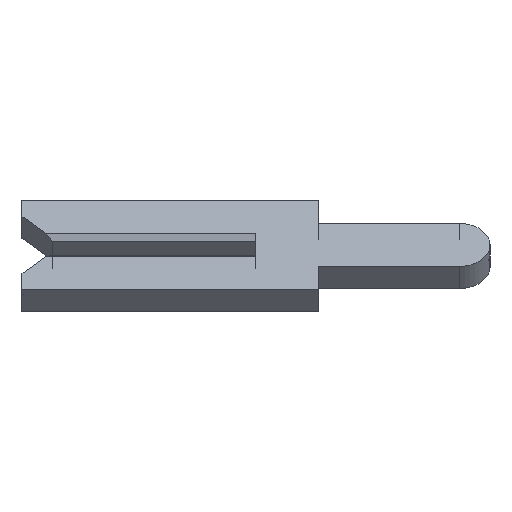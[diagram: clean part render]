
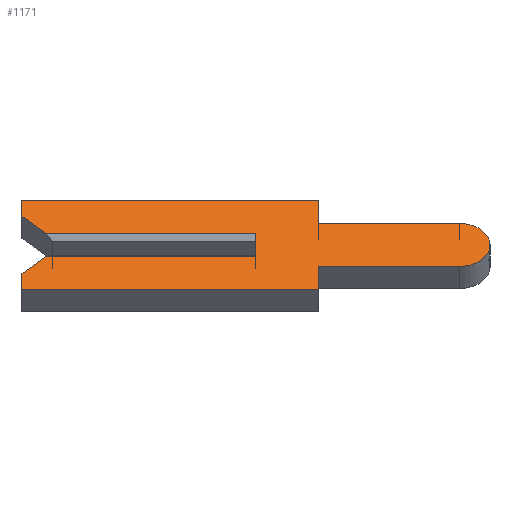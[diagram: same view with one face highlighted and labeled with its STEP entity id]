
A CAD part, left-side view. The second image highlights one B-rep face of the part: STEP entity #1171.
In plain terms, the highlighted face is planar.
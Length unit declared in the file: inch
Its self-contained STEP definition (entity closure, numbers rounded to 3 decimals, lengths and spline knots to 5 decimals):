
#3 = ORIENTED_EDGE ( 'NONE', *, *, #1020, .F. ) ;
#10 = ORIENTED_EDGE ( 'NONE', *, *, #328, .F. ) ;
#18 = DIRECTION ( 'NONE',  ( 0., -1., 0. ) ) ;
#20 = DIRECTION ( 'NONE',  ( 1., 0., 0. ) ) ;
#31 = VERTEX_POINT ( 'NONE', #914 ) ;
#44 = VECTOR ( 'NONE', #275, 39.37008 ) ;
#67 = LINE ( 'NONE', #552, #1460 ) ;
#86 = EDGE_CURVE ( 'NONE', #1322, #1650, #1158, .T. ) ;
#87 = CARTESIAN_POINT ( 'NONE',  ( -0.01, 0.15, 0.026 ) ) ;
#113 = EDGE_CURVE ( 'NONE', #359, #130, #922, .T. ) ;
#117 = VECTOR ( 'NONE', #1124, 39.37008 ) ;
#120 = VERTEX_POINT ( 'NONE', #534 ) ;
#130 = VERTEX_POINT ( 'NONE', #294 ) ;
#133 = VECTOR ( 'NONE', #931, 39.37008 ) ;
#145 = CARTESIAN_POINT ( 'NONE',  ( -0.01, 0.134, 0.01 ) ) ;
#149 = VECTOR ( 'NONE', #1108, 39.37008 ) ;
#172 = EDGE_CURVE ( 'NONE', #1380, #1164, #1426, .T. ) ;
#205 = EDGE_CURVE ( 'NONE', #312, #31, #1384, .T. ) ;
#230 = CARTESIAN_POINT ( 'NONE',  ( -0.01, 0.15, -0.04 ) ) ;
#275 = DIRECTION ( 'NONE',  ( 0., -1., 0. ) ) ;
#278 = DIRECTION ( 'NONE',  ( 0., 1., 0. ) ) ;
#294 = CARTESIAN_POINT ( 'NONE',  ( -0.01, 0., 0.01 ) ) ;
#312 = VERTEX_POINT ( 'NONE', #817 ) ;
#321 = VERTEX_POINT ( 'NONE', #949 ) ;
#328 = EDGE_CURVE ( 'NONE', #120, #1322, #1516, .T. ) ;
#333 = CARTESIAN_POINT ( 'NONE',  ( -0.01, 0.15, -0.026 ) ) ;
#359 = VERTEX_POINT ( 'NONE', #1584 ) ;
#383 = ORIENTED_EDGE ( 'NONE', *, *, #205, .F. ) ;
#388 = VECTOR ( 'NONE', #645, 39.37008 ) ;
#397 = AXIS2_PLACEMENT_3D ( 'NONE', #1318, #20, #1448 ) ;
#407 = EDGE_LOOP ( 'NONE', ( #1357, #1593, #838, #383, #664, #3, #1334, #567, #10, #1522, #1565, #471, #1489, #836 ) ) ;
#413 = CARTESIAN_POINT ( 'NONE',  ( -0.01, 0., 0.0065 ) ) ;
#426 = VECTOR ( 'NONE', #1528, 39.37008 ) ;
#471 = ORIENTED_EDGE ( 'NONE', *, *, #1507, .F. ) ;
#488 = CARTESIAN_POINT ( 'NONE',  ( -0.01, 0.1305, 0.0065 ) ) ;
#534 = CARTESIAN_POINT ( 'NONE',  ( -0.01, -0.1305, 0.0195 ) ) ;
#552 = CARTESIAN_POINT ( 'NONE',  ( -0.01, 0.15, 0.04 ) ) ;
#558 = EDGE_CURVE ( 'NONE', #1067, #312, #950, .T. ) ;
#567 = ORIENTED_EDGE ( 'NONE', *, *, #86, .F. ) ;
#627 = CARTESIAN_POINT ( 'NONE',  ( -0.01, 0.15, -0.04 ) ) ;
#645 = DIRECTION ( 'NONE',  ( 0., -1., 0. ) ) ;
#659 = CARTESIAN_POINT ( 'NONE',  ( -0.01, -0.04, 0.0195 ) ) ;
#664 = ORIENTED_EDGE ( 'NONE', *, *, #558, .F. ) ;
#671 = CARTESIAN_POINT ( 'NONE',  ( -0.01, -0.04, -0.04 ) ) ;
#684 = CARTESIAN_POINT ( 'NONE',  ( -0.01, -0.04, -0.04 ) ) ;
#731 = DIRECTION ( 'NONE',  ( 0., 0., 1. ) ) ;
#784 = DIRECTION ( 'NONE',  ( 0., 0., -1. ) ) ;
#789 = CARTESIAN_POINT ( 'NONE',  ( -0.01, 0.15, 0.04 ) ) ;
#790 = VECTOR ( 'NONE', #1268, 39.37008 ) ;
#791 = CARTESIAN_POINT ( 'NONE',  ( -0.01, -0.04, -0.0195 ) ) ;
#807 = DIRECTION ( 'NONE',  ( 0., 0., -1. ) ) ;
#816 = VECTOR ( 'NONE', #1430, 39.37008 ) ;
#817 = CARTESIAN_POINT ( 'NONE',  ( -0.01, 0.15, -0.026 ) ) ;
#818 = LINE ( 'NONE', #488, #790 ) ;
#836 = ORIENTED_EDGE ( 'NONE', *, *, #1204, .F. ) ;
#838 = ORIENTED_EDGE ( 'NONE', *, *, #1181, .F. ) ;
#879 = EDGE_CURVE ( 'NONE', #321, #1301, #1296, .T. ) ;
#914 = CARTESIAN_POINT ( 'NONE',  ( -0.01, 0.134, -0.01 ) ) ;
#922 = LINE ( 'NONE', #413, #816 ) ;
#931 = DIRECTION ( 'NONE',  ( 0., -0.707, 0.707 ) ) ;
#943 = CARTESIAN_POINT ( 'NONE',  ( -0.01, -0.04, 0.04 ) ) ;
#949 = CARTESIAN_POINT ( 'NONE',  ( -0.01, 0.15, 0.026 ) ) ;
#950 = LINE ( 'NONE', #333, #1250 ) ;
#955 = DIRECTION ( 'NONE',  ( 0., 0., -1. ) ) ;
#964 = LINE ( 'NONE', #659, #426 ) ;
#1002 = LINE ( 'NONE', #671, #1118 ) ;
#1017 = CARTESIAN_POINT ( 'NONE',  ( -0.01, -0.04, 0.0195 ) ) ;
#1020 = EDGE_CURVE ( 'NONE', #1572, #1067, #1327, .T. ) ;
#1023 = CARTESIAN_POINT ( 'NONE',  ( -0.01, -0.1305, -0.01 ) ) ;
#1054 = CARTESIAN_POINT ( 'NONE',  ( -0.01, -0.04, 0.04 ) ) ;
#1060 = LINE ( 'NONE', #1023, #388 ) ;
#1067 = VERTEX_POINT ( 'NONE', #627 ) ;
#1106 = AXIS2_PLACEMENT_3D ( 'NONE', #1419, #1403, #784 ) ;
#1108 = DIRECTION ( 'NONE',  ( 0., 0., 1. ) ) ;
#1118 = VECTOR ( 'NONE', #807, 39.37008 ) ;
#1124 = DIRECTION ( 'NONE',  ( 0., 1., 0. ) ) ;
#1127 = EDGE_CURVE ( 'NONE', #1164, #120, #964, .T. ) ;
#1147 = PLANE ( 'NONE',  #1106 ) ;
#1158 = LINE ( 'NONE', #791, #1603 ) ;
#1164 = VERTEX_POINT ( 'NONE', #1017 ) ;
#1171 = ADVANCED_FACE ( 'NONE', ( #1280 ), #1147, .F. ) ;
#1181 = EDGE_CURVE ( 'NONE', #31, #359, #1060, .T. ) ;
#1204 = EDGE_CURVE ( 'NONE', #1500, #321, #818, .T. ) ;
#1250 = VECTOR ( 'NONE', #731, 39.37008 ) ;
#1268 = DIRECTION ( 'NONE',  ( 0., 0.707, 0.707 ) ) ;
#1280 = FACE_OUTER_BOUND ( 'NONE', #407, .T. ) ;
#1296 = LINE ( 'NONE', #87, #149 ) ;
#1301 = VERTEX_POINT ( 'NONE', #789 ) ;
#1309 = CARTESIAN_POINT ( 'NONE',  ( -0.01, 0.15, 0.01 ) ) ;
#1318 = CARTESIAN_POINT ( 'NONE',  ( -0.01, -0.1305, 0. ) ) ;
#1322 = VERTEX_POINT ( 'NONE', #1413 ) ;
#1327 = LINE ( 'NONE', #230, #117 ) ;
#1334 = ORIENTED_EDGE ( 'NONE', *, *, #1560, .F. ) ;
#1357 = ORIENTED_EDGE ( 'NONE', *, *, #1423, .T. ) ;
#1380 = VERTEX_POINT ( 'NONE', #1054 ) ;
#1384 = LINE ( 'NONE', #1580, #133 ) ;
#1403 = DIRECTION ( 'NONE',  ( 1., 0., 0. ) ) ;
#1413 = CARTESIAN_POINT ( 'NONE',  ( -0.01, -0.1305, -0.0195 ) ) ;
#1419 = CARTESIAN_POINT ( 'NONE',  ( -0.01, -0.1305, 0. ) ) ;
#1423 = EDGE_CURVE ( 'NONE', #1500, #130, #1546, .T. ) ;
#1426 = LINE ( 'NONE', #943, #1566 ) ;
#1430 = DIRECTION ( 'NONE',  ( 0., 0., 1. ) ) ;
#1448 = DIRECTION ( 'NONE',  ( 0., 0., -1. ) ) ;
#1460 = VECTOR ( 'NONE', #18, 39.37008 ) ;
#1489 = ORIENTED_EDGE ( 'NONE', *, *, #879, .F. ) ;
#1500 = VERTEX_POINT ( 'NONE', #145 ) ;
#1507 = EDGE_CURVE ( 'NONE', #1301, #1380, #67, .T. ) ;
#1516 = CIRCLE ( 'NONE', #397, 0.0195 ) ;
#1522 = ORIENTED_EDGE ( 'NONE', *, *, #1127, .F. ) ;
#1528 = DIRECTION ( 'NONE',  ( 0., -1., 0. ) ) ;
#1546 = LINE ( 'NONE', #1309, #44 ) ;
#1560 = EDGE_CURVE ( 'NONE', #1650, #1572, #1002, .T. ) ;
#1565 = ORIENTED_EDGE ( 'NONE', *, *, #172, .F. ) ;
#1566 = VECTOR ( 'NONE', #955, 39.37008 ) ;
#1572 = VERTEX_POINT ( 'NONE', #684 ) ;
#1580 = CARTESIAN_POINT ( 'NONE',  ( -0.01, 0.1305, -0.0065 ) ) ;
#1584 = CARTESIAN_POINT ( 'NONE',  ( -0.01, 0., -0.01 ) ) ;
#1593 = ORIENTED_EDGE ( 'NONE', *, *, #113, .F. ) ;
#1603 = VECTOR ( 'NONE', #278, 39.37008 ) ;
#1605 = CARTESIAN_POINT ( 'NONE',  ( -0.01, -0.04, -0.0195 ) ) ;
#1650 = VERTEX_POINT ( 'NONE', #1605 ) ;
